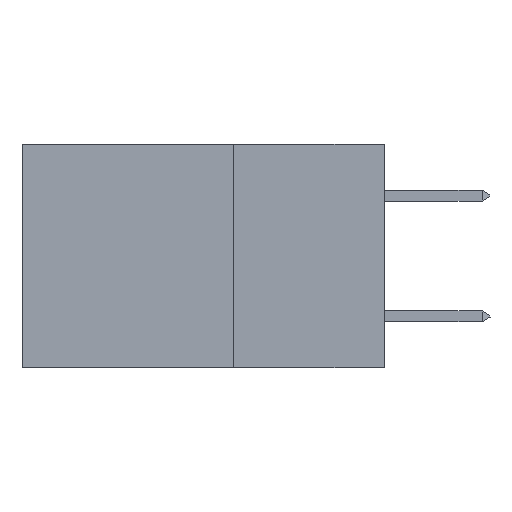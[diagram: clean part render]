
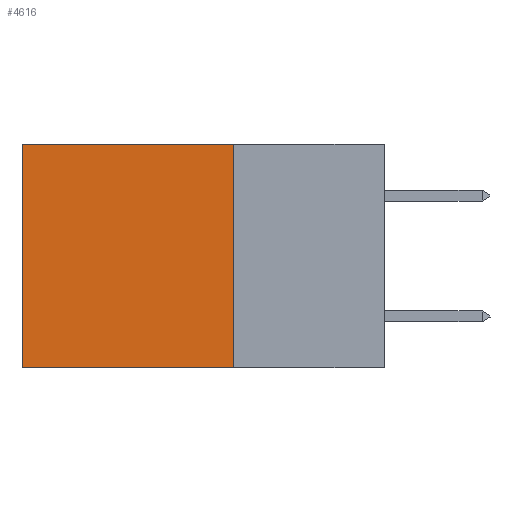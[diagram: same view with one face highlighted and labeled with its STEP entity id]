
A CAD part, left-side view. The second image highlights one B-rep face of the part: STEP entity #4616.
In plain terms, the highlighted planar face has unit normal (-1, 0, 0).
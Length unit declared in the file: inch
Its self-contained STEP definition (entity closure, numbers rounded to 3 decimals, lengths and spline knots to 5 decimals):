
#632 = CARTESIAN_POINT ( 'NONE',  ( 0.2875, 0.6, 0. ) ) ;
#1626 = VECTOR ( 'NONE', #23015, 39.37008 ) ;
#2819 = DIRECTION ( 'NONE',  ( 0., 1., 0. ) ) ;
#3082 = ORIENTED_EDGE ( 'NONE', *, *, #24725, .F. ) ;
#3378 = DIRECTION ( 'NONE',  ( 1., 0., 0. ) ) ;
#3476 = VERTEX_POINT ( 'NONE', #15936 ) ;
#4616 = ADVANCED_FACE ( 'NONE', ( #5415 ), #22097, .F. ) ;
#5415 = FACE_OUTER_BOUND ( 'NONE', #12345, .T. ) ;
#6346 = CARTESIAN_POINT ( 'NONE',  ( 0.2875, 0.25, 0. ) ) ;
#7103 = VECTOR ( 'NONE', #2819, 39.37008 ) ;
#7598 = ORIENTED_EDGE ( 'NONE', *, *, #9989, .T. ) ;
#8905 = CARTESIAN_POINT ( 'NONE',  ( 0.2875, 0.6, -0.37 ) ) ;
#8978 = DIRECTION ( 'NONE',  ( 0., 0., -1. ) ) ;
#9478 = CARTESIAN_POINT ( 'NONE',  ( 0.2875, 0.25, -0.37 ) ) ;
#9989 = EDGE_CURVE ( 'NONE', #3476, #24166, #24370, .T. ) ;
#11716 = DIRECTION ( 'NONE',  ( 0., 0., -1. ) ) ;
#11840 = AXIS2_PLACEMENT_3D ( 'NONE', #13763, #3378, #11716 ) ;
#12345 = EDGE_LOOP ( 'NONE', ( #16440, #21150, #3082, #7598 ) ) ;
#13058 = LINE ( 'NONE', #632, #21321 ) ;
#13763 = CARTESIAN_POINT ( 'NONE',  ( 0.2875, 0.25, 0. ) ) ;
#15487 = CARTESIAN_POINT ( 'NONE',  ( 0.2875, 0.25, 0. ) ) ;
#15936 = CARTESIAN_POINT ( 'NONE',  ( 0.2875, 0.25, 0. ) ) ;
#16013 = DIRECTION ( 'NONE',  ( 0., 1., 0. ) ) ;
#16149 = VERTEX_POINT ( 'NONE', #9478 ) ;
#16293 = VECTOR ( 'NONE', #16013, 39.37008 ) ;
#16440 = ORIENTED_EDGE ( 'NONE', *, *, #26573, .T. ) ;
#16452 = LINE ( 'NONE', #6346, #1626 ) ;
#19850 = EDGE_CURVE ( 'NONE', #16149, #23537, #25512, .T. ) ;
#20597 = CARTESIAN_POINT ( 'NONE',  ( 0.2875, 0.6, 0. ) ) ;
#21150 = ORIENTED_EDGE ( 'NONE', *, *, #19850, .F. ) ;
#21321 = VECTOR ( 'NONE', #8978, 39.37008 ) ;
#22097 = PLANE ( 'NONE',  #11840 ) ;
#23015 = DIRECTION ( 'NONE',  ( 0., 0., -1. ) ) ;
#23537 = VERTEX_POINT ( 'NONE', #8905 ) ;
#23590 = CARTESIAN_POINT ( 'NONE',  ( 0.2875, 0.25, -0.37 ) ) ;
#24166 = VERTEX_POINT ( 'NONE', #20597 ) ;
#24370 = LINE ( 'NONE', #15487, #16293 ) ;
#24725 = EDGE_CURVE ( 'NONE', #3476, #16149, #16452, .T. ) ;
#25512 = LINE ( 'NONE', #23590, #7103 ) ;
#26573 = EDGE_CURVE ( 'NONE', #24166, #23537, #13058, .T. ) ;
